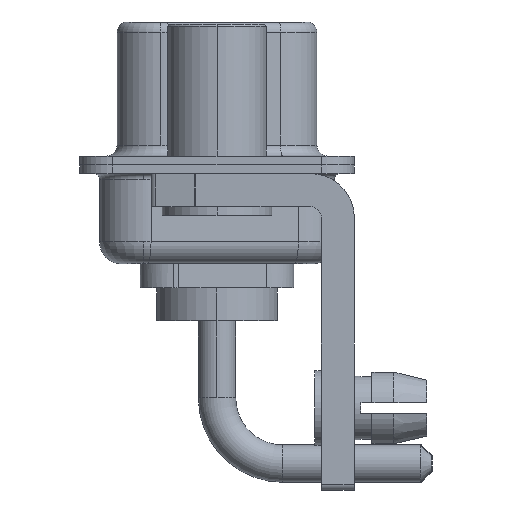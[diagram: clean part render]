
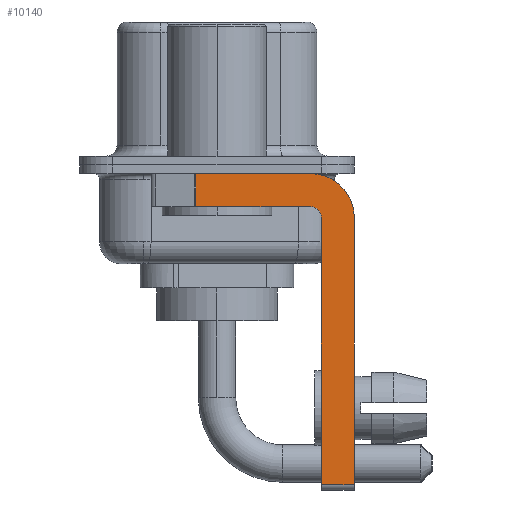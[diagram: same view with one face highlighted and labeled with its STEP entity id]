
A CAD part, left-side view. The second image highlights one B-rep face of the part: STEP entity #10140.
In plain terms, the highlighted planar face has unit normal (-1, 0, 0).
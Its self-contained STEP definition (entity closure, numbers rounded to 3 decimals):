
#698 = VECTOR ( 'NONE', #5210, 1000. ) ;
#1093 = DIRECTION ( 'NONE',  ( 0., -1., 0. ) ) ;
#1446 = ORIENTED_EDGE ( 'NONE', *, *, #2805, .F. ) ;
#1489 = CARTESIAN_POINT ( 'NONE',  ( -2.9, 0.978, -1.9 ) ) ;
#1552 = LINE ( 'NONE', #12611, #2626 ) ;
#1708 = DIRECTION ( 'NONE',  ( 0., 0., -1. ) ) ;
#1969 = VERTEX_POINT ( 'NONE', #16699 ) ;
#2307 = VERTEX_POINT ( 'NONE', #13603 ) ;
#2626 = VECTOR ( 'NONE', #7093, 1000. ) ;
#2642 = LINE ( 'NONE', #4351, #3653 ) ;
#2660 = LINE ( 'NONE', #3827, #698 ) ;
#2805 = EDGE_CURVE ( 'NONE', #14318, #14935, #6516, .T. ) ;
#2807 = LINE ( 'NONE', #5799, #16856 ) ;
#2942 = EDGE_CURVE ( 'NONE', #12923, #10439, #2807, .T. ) ;
#3500 = EDGE_CURVE ( 'NONE', #2307, #14318, #9977, .T. ) ;
#3505 = DIRECTION ( 'NONE',  ( 1., 0., 0. ) ) ;
#3565 = CARTESIAN_POINT ( 'NONE',  ( -2.9, -4.75, -14.55 ) ) ;
#3626 = CARTESIAN_POINT ( 'NONE',  ( -2.9, -4.25, -2.4 ) ) ;
#3653 = VECTOR ( 'NONE', #12494, 1000. ) ;
#3827 = CARTESIAN_POINT ( 'NONE',  ( -2.9, 0.978, -1.9 ) ) ;
#3886 = VERTEX_POINT ( 'NONE', #3565 ) ;
#4028 = EDGE_CURVE ( 'NONE', #7571, #10439, #2660, .T. ) ;
#4351 = CARTESIAN_POINT ( 'NONE',  ( -2.9, 3., -0.4 ) ) ;
#4857 = ORIENTED_EDGE ( 'NONE', *, *, #2942, .F. ) ;
#4872 = DIRECTION ( 'NONE',  ( 0., 0., -1. ) ) ;
#4964 = CARTESIAN_POINT ( 'NONE',  ( -2.9, -4.25, -2.4 ) ) ;
#5107 = EDGE_LOOP ( 'NONE', ( #8377, #8006, #4857, #11036, #14090, #12554, #1446, #5487 ) ) ;
#5210 = DIRECTION ( 'NONE',  ( 0., 0., -1. ) ) ;
#5402 = AXIS2_PLACEMENT_3D ( 'NONE', #4964, #3505, #4872 ) ;
#5487 = ORIENTED_EDGE ( 'NONE', *, *, #3500, .F. ) ;
#5524 = DIRECTION ( 'NONE',  ( 0., 1., 0. ) ) ;
#5799 = CARTESIAN_POINT ( 'NONE',  ( -2.9, -4.25, -1.9 ) ) ;
#6145 = CIRCLE ( 'NONE', #17130, 0.5 ) ;
#6516 = LINE ( 'NONE', #16206, #7034 ) ;
#6636 = LINE ( 'NONE', #10716, #6899 ) ;
#6657 = DIRECTION ( 'NONE',  ( 0., 0., -1. ) ) ;
#6709 = DIRECTION ( 'NONE',  ( 0., 0., 1. ) ) ;
#6899 = VECTOR ( 'NONE', #1093, 1000. ) ;
#7034 = VECTOR ( 'NONE', #1708, 1000. ) ;
#7093 = DIRECTION ( 'NONE',  ( 0., 0., 1. ) ) ;
#7571 = VERTEX_POINT ( 'NONE', #14751 ) ;
#7667 = FACE_OUTER_BOUND ( 'NONE', #5107, .T. ) ;
#8006 = ORIENTED_EDGE ( 'NONE', *, *, #4028, .T. ) ;
#8377 = ORIENTED_EDGE ( 'NONE', *, *, #11980, .F. ) ;
#8843 = EDGE_CURVE ( 'NONE', #3886, #1969, #1552, .T. ) ;
#9167 = DIRECTION ( 'NONE',  ( -1., 0., 0. ) ) ;
#9288 = EDGE_CURVE ( 'NONE', #1969, #12923, #6145, .T. ) ;
#9899 = CARTESIAN_POINT ( 'NONE',  ( -2.9, -4.25, -1.9 ) ) ;
#9977 = CIRCLE ( 'NONE', #10551, 2. ) ;
#10140 = ADVANCED_FACE ( 'NONE', ( #7667 ), #11645, .F. ) ;
#10182 = CARTESIAN_POINT ( 'NONE',  ( -2.9, -6.25, -14.55 ) ) ;
#10439 = VERTEX_POINT ( 'NONE', #1489 ) ;
#10551 = AXIS2_PLACEMENT_3D ( 'NONE', #17886, #16607, #6657 ) ;
#10716 = CARTESIAN_POINT ( 'NONE',  ( -2.9, -4.25, -14.55 ) ) ;
#11036 = ORIENTED_EDGE ( 'NONE', *, *, #9288, .F. ) ;
#11645 = PLANE ( 'NONE',  #5402 ) ;
#11980 = EDGE_CURVE ( 'NONE', #7571, #2307, #2642, .T. ) ;
#12494 = DIRECTION ( 'NONE',  ( 0., -1., 0. ) ) ;
#12554 = ORIENTED_EDGE ( 'NONE', *, *, #16627, .T. ) ;
#12611 = CARTESIAN_POINT ( 'NONE',  ( -2.9, -4.75, -14.8 ) ) ;
#12923 = VERTEX_POINT ( 'NONE', #9899 ) ;
#13603 = CARTESIAN_POINT ( 'NONE',  ( -2.9, -4.25, -0.4 ) ) ;
#14090 = ORIENTED_EDGE ( 'NONE', *, *, #8843, .F. ) ;
#14318 = VERTEX_POINT ( 'NONE', #15166 ) ;
#14751 = CARTESIAN_POINT ( 'NONE',  ( -2.9, 0.978, -0.4 ) ) ;
#14935 = VERTEX_POINT ( 'NONE', #10182 ) ;
#15166 = CARTESIAN_POINT ( 'NONE',  ( -2.9, -6.25, -2.4 ) ) ;
#16206 = CARTESIAN_POINT ( 'NONE',  ( -2.9, -6.25, -2.4 ) ) ;
#16607 = DIRECTION ( 'NONE',  ( 1., 0., 0. ) ) ;
#16627 = EDGE_CURVE ( 'NONE', #3886, #14935, #6636, .T. ) ;
#16699 = CARTESIAN_POINT ( 'NONE',  ( -2.9, -4.75, -2.4 ) ) ;
#16856 = VECTOR ( 'NONE', #5524, 1000. ) ;
#17130 = AXIS2_PLACEMENT_3D ( 'NONE', #3626, #9167, #6709 ) ;
#17886 = CARTESIAN_POINT ( 'NONE',  ( -2.9, -4.25, -2.4 ) ) ;
